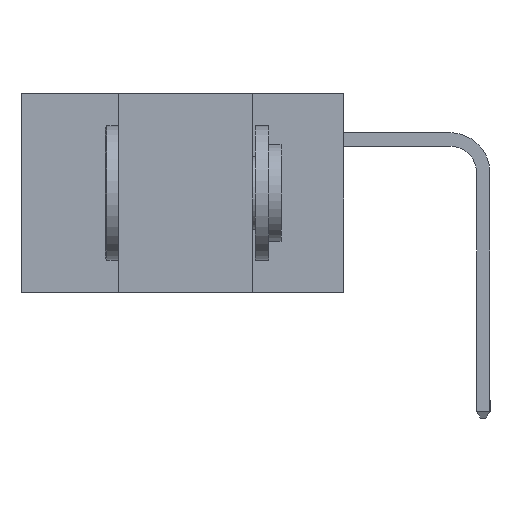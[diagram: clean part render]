
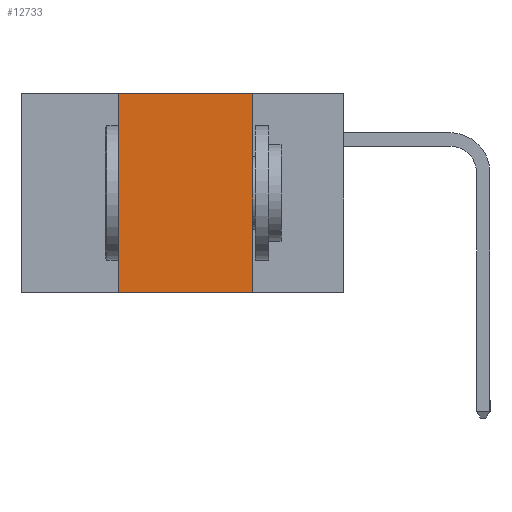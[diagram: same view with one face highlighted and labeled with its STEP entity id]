
A CAD part, left-side view. The second image highlights one B-rep face of the part: STEP entity #12733.
In plain terms, the highlighted planar face has unit normal (-1, 0, 0).
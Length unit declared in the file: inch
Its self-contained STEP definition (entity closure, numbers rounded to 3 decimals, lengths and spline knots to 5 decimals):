
#21 = VERTEX_POINT ( 'NONE', #7668 ) ;
#222 = VERTEX_POINT ( 'NONE', #12567 ) ;
#482 = DIRECTION ( 'NONE',  ( 0., -1., 0. ) ) ;
#838 = DIRECTION ( 'NONE',  ( 0., 0., -1. ) ) ;
#1001 = VECTOR ( 'NONE', #12103, 39.37008 ) ;
#1277 = LINE ( 'NONE', #15776, #8052 ) ;
#2517 = VECTOR ( 'NONE', #11916, 39.37008 ) ;
#4161 = CARTESIAN_POINT ( 'NONE',  ( 0., 0.42, -0.37 ) ) ;
#4378 = CARTESIAN_POINT ( 'NONE',  ( 0., 0.6, 0. ) ) ;
#4593 = VECTOR ( 'NONE', #838, 39.37008 ) ;
#4849 = ORIENTED_EDGE ( 'NONE', *, *, #10745, .F. ) ;
#6090 = PLANE ( 'NONE',  #14295 ) ;
#6154 = DIRECTION ( 'NONE',  ( 1., 0., 0. ) ) ;
#6271 = CARTESIAN_POINT ( 'NONE',  ( 0., 0.17, -0.37 ) ) ;
#6599 = ORIENTED_EDGE ( 'NONE', *, *, #9911, .F. ) ;
#7668 = CARTESIAN_POINT ( 'NONE',  ( 0., 0.17, 0. ) ) ;
#8052 = VECTOR ( 'NONE', #482, 39.37008 ) ;
#8107 = EDGE_LOOP ( 'NONE', ( #4849, #6599, #9248, #11562 ) ) ;
#8188 = LINE ( 'NONE', #4378, #1001 ) ;
#8195 = EDGE_CURVE ( 'NONE', #222, #13892, #1277, .T. ) ;
#9040 = EDGE_CURVE ( 'NONE', #222, #10176, #15275, .T. ) ;
#9070 = CARTESIAN_POINT ( 'NONE',  ( 0., 0.42, 0. ) ) ;
#9248 = ORIENTED_EDGE ( 'NONE', *, *, #9040, .F. ) ;
#9911 = EDGE_CURVE ( 'NONE', #10176, #21, #8188, .T. ) ;
#10176 = VERTEX_POINT ( 'NONE', #9070 ) ;
#10745 = EDGE_CURVE ( 'NONE', #21, #13892, #14674, .T. ) ;
#11248 = CARTESIAN_POINT ( 'NONE',  ( 0., 0.6, 0. ) ) ;
#11562 = ORIENTED_EDGE ( 'NONE', *, *, #8195, .T. ) ;
#11643 = FACE_OUTER_BOUND ( 'NONE', #8107, .T. ) ;
#11916 = DIRECTION ( 'NONE',  ( 0., 0., 1. ) ) ;
#12103 = DIRECTION ( 'NONE',  ( 0., -1., 0. ) ) ;
#12567 = CARTESIAN_POINT ( 'NONE',  ( 0., 0.42, -0.37 ) ) ;
#12733 = ADVANCED_FACE ( 'NONE', ( #11643 ), #6090, .F. ) ;
#13892 = VERTEX_POINT ( 'NONE', #14558 ) ;
#14295 = AXIS2_PLACEMENT_3D ( 'NONE', #11248, #6154, #14839 ) ;
#14558 = CARTESIAN_POINT ( 'NONE',  ( 0., 0.17, -0.37 ) ) ;
#14674 = LINE ( 'NONE', #6271, #4593 ) ;
#14839 = DIRECTION ( 'NONE',  ( 0., 0., -1. ) ) ;
#15275 = LINE ( 'NONE', #4161, #2517 ) ;
#15776 = CARTESIAN_POINT ( 'NONE',  ( 0., 0.6, -0.37 ) ) ;
